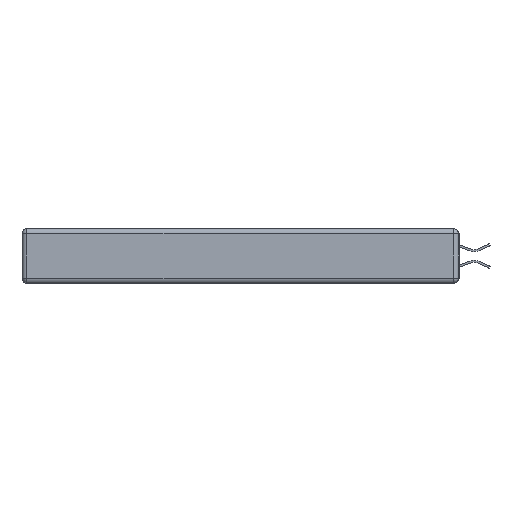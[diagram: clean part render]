
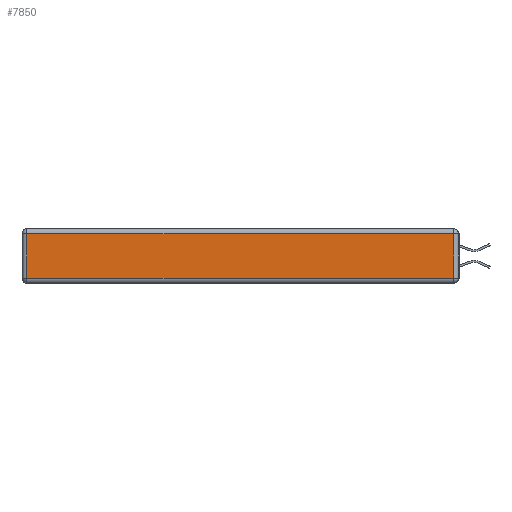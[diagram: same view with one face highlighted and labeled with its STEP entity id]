
A CAD part, left-side view. The second image highlights one B-rep face of the part: STEP entity #7850.
In plain terms, the highlighted planar face has unit normal (-1, 0, 0).
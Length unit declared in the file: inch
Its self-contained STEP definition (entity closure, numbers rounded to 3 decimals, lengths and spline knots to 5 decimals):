
#153 = CARTESIAN_POINT ( 'NONE',  ( 0., 2.75, -0.03 ) ) ;
#305 = PLANE ( 'NONE',  #17127 ) ;
#388 = CARTESIAN_POINT ( 'NONE',  ( 0., 0.03, -0.03 ) ) ;
#1698 = ORIENTED_EDGE ( 'NONE', *, *, #11025, .T. ) ;
#1873 = DIRECTION ( 'NONE',  ( 0., 0., -1. ) ) ;
#2448 = VERTEX_POINT ( 'NONE', #6571 ) ;
#4146 = ORIENTED_EDGE ( 'NONE', *, *, #8539, .T. ) ;
#4738 = LINE ( 'NONE', #17438, #4979 ) ;
#4979 = VECTOR ( 'NONE', #1873, 39.37008 ) ;
#6019 = CARTESIAN_POINT ( 'NONE',  ( 0., 0.03, -0.343 ) ) ;
#6571 = CARTESIAN_POINT ( 'NONE',  ( 0., 2.72, -0.313 ) ) ;
#6612 = EDGE_CURVE ( 'NONE', #2448, #7897, #7115, .T. ) ;
#7115 = LINE ( 'NONE', #7374, #17767 ) ;
#7374 = CARTESIAN_POINT ( 'NONE',  ( 0., 0., -0.313 ) ) ;
#7586 = DIRECTION ( 'NONE',  ( 0., 0., 1. ) ) ;
#7850 = ADVANCED_FACE ( 'NONE', ( #11831 ), #305, .T. ) ;
#7897 = VERTEX_POINT ( 'NONE', #13287 ) ;
#8282 = VERTEX_POINT ( 'NONE', #388 ) ;
#8539 = EDGE_CURVE ( 'NONE', #7897, #8282, #20015, .T. ) ;
#8961 = DIRECTION ( 'NONE',  ( 0., -1., 0. ) ) ;
#9055 = EDGE_LOOP ( 'NONE', ( #19524, #4146, #10295, #1698 ) ) ;
#9243 = DIRECTION ( 'NONE',  ( -1., 0., 0. ) ) ;
#9309 = VECTOR ( 'NONE', #7586, 39.37008 ) ;
#10295 = ORIENTED_EDGE ( 'NONE', *, *, #15149, .T. ) ;
#11025 = EDGE_CURVE ( 'NONE', #18363, #2448, #4738, .T. ) ;
#11831 = FACE_OUTER_BOUND ( 'NONE', #9055, .T. ) ;
#13287 = CARTESIAN_POINT ( 'NONE',  ( 0., 0.03, -0.313 ) ) ;
#14202 = DIRECTION ( 'NONE',  ( 0., 1., 0. ) ) ;
#14382 = DIRECTION ( 'NONE',  ( 0., 0., 1. ) ) ;
#14596 = CARTESIAN_POINT ( 'NONE',  ( 0., 0., -0.343 ) ) ;
#15149 = EDGE_CURVE ( 'NONE', #8282, #18363, #15653, .T. ) ;
#15653 = LINE ( 'NONE', #153, #19401 ) ;
#16666 = CARTESIAN_POINT ( 'NONE',  ( 0., 2.72, -0.03 ) ) ;
#17127 = AXIS2_PLACEMENT_3D ( 'NONE', #14596, #9243, #14382 ) ;
#17438 = CARTESIAN_POINT ( 'NONE',  ( 0., 2.72, -0.343 ) ) ;
#17767 = VECTOR ( 'NONE', #8961, 39.37008 ) ;
#18363 = VERTEX_POINT ( 'NONE', #16666 ) ;
#19401 = VECTOR ( 'NONE', #14202, 39.37008 ) ;
#19524 = ORIENTED_EDGE ( 'NONE', *, *, #6612, .T. ) ;
#20015 = LINE ( 'NONE', #6019, #9309 ) ;
